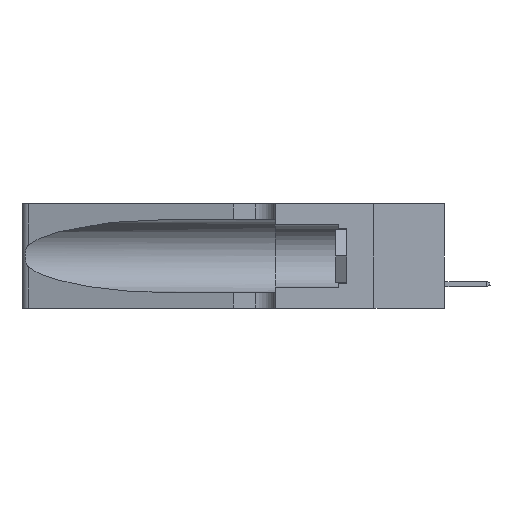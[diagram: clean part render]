
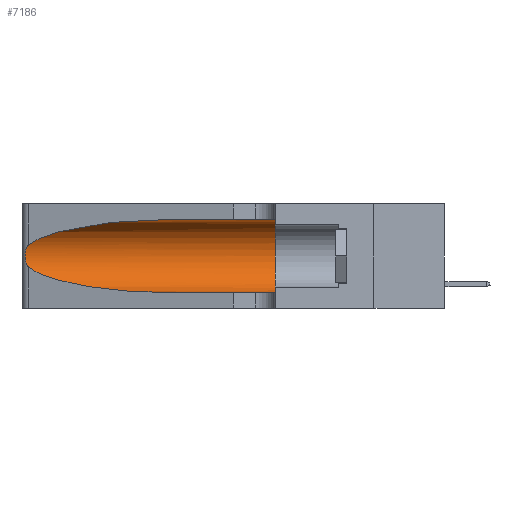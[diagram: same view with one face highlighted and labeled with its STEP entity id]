
A CAD part, left-side view. The second image highlights one B-rep face of the part: STEP entity #7186.
In plain terms, the highlighted cylindrical face has radius 3.308 mm (diameter 6.617 mm), a partial arc.
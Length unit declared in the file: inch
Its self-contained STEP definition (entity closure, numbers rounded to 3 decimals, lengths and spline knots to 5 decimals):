
#93 = DIRECTION ( 'NONE',  ( 0., 1., 0. ) ) ;
#259 = CARTESIAN_POINT ( 'NONE',  ( 0.1305, 0.35, 0.185 ) ) ;
#372 = CARTESIAN_POINT ( 'NONE',  ( 0.25787, 1.23484, 0.2124 ) ) ;
#650 = CARTESIAN_POINT ( 'NONE',  ( 0.25487, 1.22718, 0.14631 ) ) ;
#2104 = DIRECTION ( 'NONE',  ( 0., -1., 0. ) ) ;
#2437 = CARTESIAN_POINT ( 'NONE',  ( 0.2373, 1.15595, 0.08982 ) ) ;
#2601 = VECTOR ( 'NONE', #9282, 39.37008 ) ;
#2709 = B_SPLINE_CURVE_WITH_KNOTS ( 'NONE', 3,
 ( #7343, #4699, #8311, #372, #13946, #8603, #7402, #16642, #4346, #14921, #9601, #13587, #16699, #650 ),
 .UNSPECIFIED., .F., .F.,
 ( 4, 2, 2, 2, 2, 2, 4 ),
 ( 0., 0.00027, 0.00053, 0.00107, 0.0016, 0.00187, 0.00214 ),
 .UNSPECIFIED. ) ;
#2788 = CYLINDRICAL_SURFACE ( 'NONE', #9962, 0.13025 ) ;
#2894 = CARTESIAN_POINT ( 'NONE',  ( 0.1305, 1.61858, 0.31525 ) ) ;
#2935 = CARTESIAN_POINT ( 'NONE',  ( 0.25487, 1.22718, 0.14631 ) ) ;
#3133 = ORIENTED_EDGE ( 'NONE', *, *, #7829, .F. ) ;
#3689 = VERTEX_POINT ( 'NONE', #15423 ) ;
#4128 = DIRECTION ( 'NONE',  ( 0., 0., 1. ) ) ;
#4224 = DIRECTION ( 'NONE',  ( 0., -1., 0. ) ) ;
#4318 = EDGE_CURVE ( 'NONE', #12784, #5900, #11721, .T. ) ;
#4346 = CARTESIAN_POINT ( 'NONE',  ( 0.26017, 1.23833, 0.17102 ) ) ;
#4370 = CARTESIAN_POINT ( 'NONE',  ( 0.2373, 1.15595, 0.28018 ) ) ;
#4699 = CARTESIAN_POINT ( 'NONE',  ( 0.25555, 1.22994, 0.2215 ) ) ;
#4822 = CARTESIAN_POINT ( 'NONE',  ( 0.1305, 1.61858, 0.185 ) ) ;
#5196 = EDGE_LOOP ( 'NONE', ( #8029, #9263, #5805, #6805, #13696, #3133 ) ) ;
#5365 = CARTESIAN_POINT ( 'NONE',  ( 0.1305, 1.61858, 0.05475 ) ) ;
#5727 = CARTESIAN_POINT ( 'NONE',  ( 0.1305, 0.72297, 0.31525 ) ) ;
#5805 = ORIENTED_EDGE ( 'NONE', *, *, #4318, .T. ) ;
#5900 = VERTEX_POINT ( 'NONE', #10357 ) ;
#6805 = ORIENTED_EDGE ( 'NONE', *, *, #17030, .T. ) ;
#6958 = EDGE_CURVE ( 'NONE', #13948, #3689, #11089, .T. ) ;
#7186 = ADVANCED_FACE ( 'NONE', ( #16677 ), #2788, .F. ) ;
#7240 = CARTESIAN_POINT ( 'NONE',  ( 0.1305, 0.72297, 0.31525 ) ) ;
#7343 = CARTESIAN_POINT ( 'NONE',  ( 0.25487, 1.22718, 0.22369 ) ) ;
#7345 = VECTOR ( 'NONE', #4224, 39.37008 ) ;
#7402 = CARTESIAN_POINT ( 'NONE',  ( 0.26075, 1.23896, 0.19203 ) ) ;
#7632 = CARTESIAN_POINT ( 'NONE',  ( 0.18966, 0.96281, 0.05475 ) ) ;
#7829 = EDGE_CURVE ( 'NONE', #14637, #13948, #13493, .T. ) ;
#8029 = ORIENTED_EDGE ( 'NONE', *, *, #14590, .T. ) ;
#8311 = CARTESIAN_POINT ( 'NONE',  ( 0.25639, 1.23184, 0.21858 ) ) ;
#8603 = CARTESIAN_POINT ( 'NONE',  ( 0.26018, 1.23835, 0.19895 ) ) ;
#8671 = CARTESIAN_POINT ( 'NONE',  ( 0.25487, 1.22718, 0.22369 ) ) ;
#9263 = ORIENTED_EDGE ( 'NONE', *, *, #13501, .T. ) ;
#9282 = DIRECTION ( 'NONE',  ( 0., -1., 0. ) ) ;
#9594 = CARTESIAN_POINT ( 'NONE',  ( 0.1305, 0.35, 0.31525 ) ) ;
#9601 = CARTESIAN_POINT ( 'NONE',  ( 0.25789, 1.23486, 0.15765 ) ) ;
#9962 = AXIS2_PLACEMENT_3D ( 'NONE', #4822, #2104, #11248 ) ;
#9966 = VERTEX_POINT ( 'NONE', #8671 ) ;
#10035 = LINE ( 'NONE', #5365, #2601 ) ;
#10208 = AXIS2_PLACEMENT_3D ( 'NONE', #259, #93, #4128 ) ;
#10357 = CARTESIAN_POINT ( 'NONE',  ( 0.1305, 0.72297, 0.05475 ) ) ;
#10795 = CARTESIAN_POINT ( 'NONE',  ( 0.25487, 1.22718, 0.22369 ) ) ;
#11089 = CIRCLE ( 'NONE', #10208, 0.13025 ) ;
#11248 = DIRECTION ( 'NONE',  ( 0., 0., -1. ) ) ;
#11721 =( BOUNDED_CURVE ( )  B_SPLINE_CURVE ( 3, ( #15733, #2437, #7632, #14285 ),
 .UNSPECIFIED., .F., .F. ) 
 B_SPLINE_CURVE_WITH_KNOTS ( ( 4, 4 ),
 ( 3.44316, 4.71239 ),
 .UNSPECIFIED. ) 
 CURVE ( )  GEOMETRIC_REPRESENTATION_ITEM ( )  RATIONAL_B_SPLINE_CURVE ( ( 1., 0.87, 0.87, 1. ) ) 
 REPRESENTATION_ITEM ( '' )  );
#12298 = CARTESIAN_POINT ( 'NONE',  ( 0.18966, 0.96281, 0.31525 ) ) ;
#12784 = VERTEX_POINT ( 'NONE', #2935 ) ;
#13493 = LINE ( 'NONE', #2894, #7345 ) ;
#13501 = EDGE_CURVE ( 'NONE', #9966, #12784, #2709, .T. ) ;
#13587 = CARTESIAN_POINT ( 'NONE',  ( 0.25639, 1.23186, 0.15144 ) ) ;
#13696 = ORIENTED_EDGE ( 'NONE', *, *, #6958, .F. ) ;
#13946 = CARTESIAN_POINT ( 'NONE',  ( 0.25854, 1.2359, 0.20912 ) ) ;
#13948 = VERTEX_POINT ( 'NONE', #9594 ) ;
#14285 = CARTESIAN_POINT ( 'NONE',  ( 0.1305, 0.72297, 0.05475 ) ) ;
#14590 = EDGE_CURVE ( 'NONE', #14637, #9966, #17145, .T. ) ;
#14637 = VERTEX_POINT ( 'NONE', #7240 ) ;
#14921 = CARTESIAN_POINT ( 'NONE',  ( 0.25856, 1.23593, 0.16098 ) ) ;
#15423 = CARTESIAN_POINT ( 'NONE',  ( 0.1305, 0.35, 0.05475 ) ) ;
#15733 = CARTESIAN_POINT ( 'NONE',  ( 0.25487, 1.22718, 0.14631 ) ) ;
#16642 = CARTESIAN_POINT ( 'NONE',  ( 0.26075, 1.23896, 0.178 ) ) ;
#16677 = FACE_OUTER_BOUND ( 'NONE', #5196, .T. ) ;
#16699 = CARTESIAN_POINT ( 'NONE',  ( 0.25555, 1.22993, 0.14849 ) ) ;
#17030 = EDGE_CURVE ( 'NONE', #5900, #3689, #10035, .T. ) ;
#17145 =( BOUNDED_CURVE ( )  B_SPLINE_CURVE ( 3, ( #5727, #12298, #4370, #10795 ),
 .UNSPECIFIED., .F., .T. ) 
 B_SPLINE_CURVE_WITH_KNOTS ( ( 4, 4 ),
 ( 1.5708, 2.84003 ),
 .UNSPECIFIED. ) 
 CURVE ( )  GEOMETRIC_REPRESENTATION_ITEM ( )  RATIONAL_B_SPLINE_CURVE ( ( 1., 0.87, 0.87, 1. ) ) 
 REPRESENTATION_ITEM ( '' )  );
